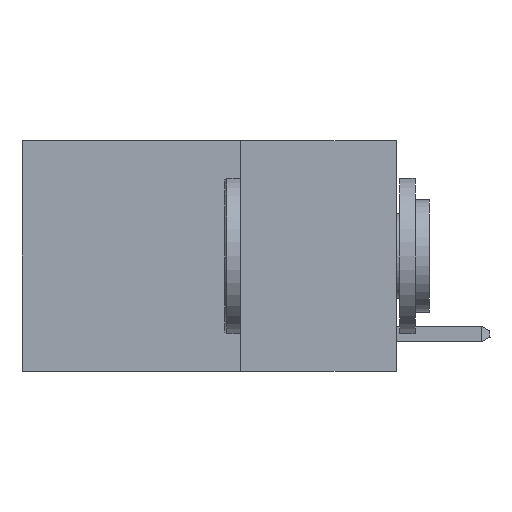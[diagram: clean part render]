
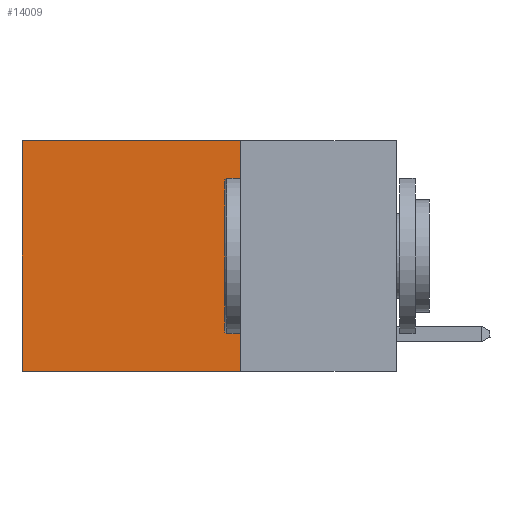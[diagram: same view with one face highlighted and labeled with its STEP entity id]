
A CAD part, left-side view. The second image highlights one B-rep face of the part: STEP entity #14009.
In plain terms, the highlighted planar face has unit normal (-1, 0, 0).
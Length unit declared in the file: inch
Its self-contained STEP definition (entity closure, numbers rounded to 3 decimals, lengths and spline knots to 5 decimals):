
#1206 = AXIS2_PLACEMENT_3D ( 'NONE', #3870, #8052, #21020 ) ;
#1250 = ORIENTED_EDGE ( 'NONE', *, *, #4712, .F. ) ;
#1303 = CARTESIAN_POINT ( 'NONE',  ( 0.2625, 0.25, 0. ) ) ;
#1666 = DIRECTION ( 'NONE',  ( 0., 0., -1. ) ) ;
#3736 = CARTESIAN_POINT ( 'NONE',  ( 0.2625, 0.6, -0.37 ) ) ;
#3870 = CARTESIAN_POINT ( 'NONE',  ( 0.2625, 0.25, 0. ) ) ;
#4268 = CARTESIAN_POINT ( 'NONE',  ( 0.2625, 0.6, 0. ) ) ;
#4712 = EDGE_CURVE ( 'NONE', #10673, #16986, #14915, .T. ) ;
#4862 = VECTOR ( 'NONE', #23891, 39.37008 ) ;
#5698 = ORIENTED_EDGE ( 'NONE', *, *, #15786, .F. ) ;
#5801 = PLANE ( 'NONE',  #1206 ) ;
#6625 = VERTEX_POINT ( 'NONE', #18985 ) ;
#8052 = DIRECTION ( 'NONE',  ( 1., 0., 0. ) ) ;
#9129 = CARTESIAN_POINT ( 'NONE',  ( 0.2625, 0.25, -0.37 ) ) ;
#9490 = LINE ( 'NONE', #24069, #13893 ) ;
#10673 = VERTEX_POINT ( 'NONE', #13168 ) ;
#11331 = ORIENTED_EDGE ( 'NONE', *, *, #14362, .T. ) ;
#11906 = DIRECTION ( 'NONE',  ( 0., 0., -1. ) ) ;
#12243 = VERTEX_POINT ( 'NONE', #4268 ) ;
#12757 = DIRECTION ( 'NONE',  ( 0., 1., 0. ) ) ;
#13168 = CARTESIAN_POINT ( 'NONE',  ( 0.2625, 0.25, -0.37 ) ) ;
#13893 = VECTOR ( 'NONE', #1666, 39.37008 ) ;
#14009 = ADVANCED_FACE ( 'NONE', ( #16251 ), #5801, .F. ) ;
#14092 = EDGE_LOOP ( 'NONE', ( #20332, #1250, #5698, #11331 ) ) ;
#14362 = EDGE_CURVE ( 'NONE', #6625, #12243, #15406, .T. ) ;
#14915 = LINE ( 'NONE', #9129, #4862 ) ;
#15406 = LINE ( 'NONE', #1303, #17942 ) ;
#15786 = EDGE_CURVE ( 'NONE', #6625, #10673, #9490, .T. ) ;
#16251 = FACE_OUTER_BOUND ( 'NONE', #14092, .T. ) ;
#16278 = VECTOR ( 'NONE', #11906, 39.37008 ) ;
#16986 = VERTEX_POINT ( 'NONE', #3736 ) ;
#17942 = VECTOR ( 'NONE', #12757, 39.37008 ) ;
#18583 = LINE ( 'NONE', #22873, #16278 ) ;
#18985 = CARTESIAN_POINT ( 'NONE',  ( 0.2625, 0.25, 0. ) ) ;
#20332 = ORIENTED_EDGE ( 'NONE', *, *, #24302, .T. ) ;
#21020 = DIRECTION ( 'NONE',  ( 0., 0., -1. ) ) ;
#22873 = CARTESIAN_POINT ( 'NONE',  ( 0.2625, 0.6, 0. ) ) ;
#23891 = DIRECTION ( 'NONE',  ( 0., 1., 0. ) ) ;
#24069 = CARTESIAN_POINT ( 'NONE',  ( 0.2625, 0.25, 0. ) ) ;
#24302 = EDGE_CURVE ( 'NONE', #12243, #16986, #18583, .T. ) ;
